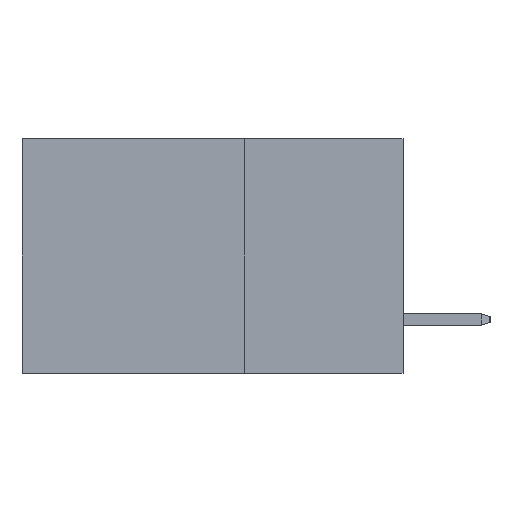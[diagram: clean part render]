
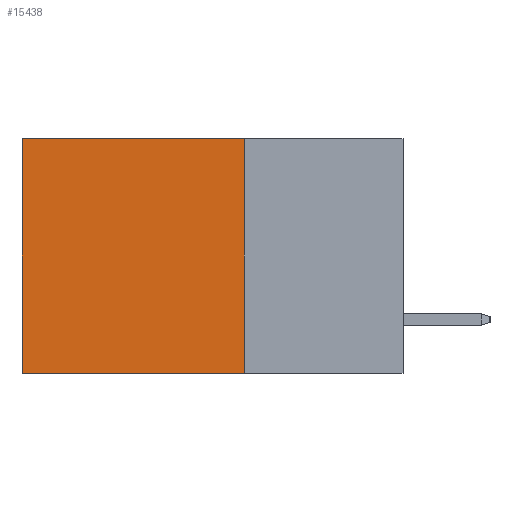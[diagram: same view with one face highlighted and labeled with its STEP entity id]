
A CAD part, left-side view. The second image highlights one B-rep face of the part: STEP entity #15438.
In plain terms, the highlighted planar face has unit normal (-1, 0, 0).
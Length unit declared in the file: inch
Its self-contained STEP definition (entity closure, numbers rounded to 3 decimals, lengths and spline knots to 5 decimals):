
#345 = VERTEX_POINT ( 'NONE', #10332 ) ;
#437 = DIRECTION ( 'NONE',  ( 0., 1., 0. ) ) ;
#1494 = CARTESIAN_POINT ( 'NONE',  ( 0.2875, 0.6, 0. ) ) ;
#1544 = CARTESIAN_POINT ( 'NONE',  ( 0.2875, 0.25, -0.37 ) ) ;
#1987 = VERTEX_POINT ( 'NONE', #7854 ) ;
#2152 = AXIS2_PLACEMENT_3D ( 'NONE', #7720, #12922, #12130 ) ;
#2515 = PLANE ( 'NONE',  #2152 ) ;
#2656 = VERTEX_POINT ( 'NONE', #9870 ) ;
#4456 = LINE ( 'NONE', #1544, #7580 ) ;
#4631 = EDGE_CURVE ( 'NONE', #1987, #2656, #4456, .T. ) ;
#4733 = EDGE_CURVE ( 'NONE', #345, #10092, #6666, .T. ) ;
#5535 = VECTOR ( 'NONE', #11903, 39.37008 ) ;
#5857 = DIRECTION ( 'NONE',  ( 0., 0., -1. ) ) ;
#5932 = EDGE_CURVE ( 'NONE', #345, #1987, #12083, .T. ) ;
#6666 = LINE ( 'NONE', #15775, #7291 ) ;
#7291 = VECTOR ( 'NONE', #8117, 39.37008 ) ;
#7580 = VECTOR ( 'NONE', #437, 39.37008 ) ;
#7720 = CARTESIAN_POINT ( 'NONE',  ( 0.2875, 0.25, 0. ) ) ;
#7854 = CARTESIAN_POINT ( 'NONE',  ( 0.2875, 0.25, -0.37 ) ) ;
#8117 = DIRECTION ( 'NONE',  ( 0., 1., 0. ) ) ;
#8419 = CARTESIAN_POINT ( 'NONE',  ( 0.2875, 0.25, 0. ) ) ;
#8992 = FACE_OUTER_BOUND ( 'NONE', #11119, .T. ) ;
#9450 = ORIENTED_EDGE ( 'NONE', *, *, #4733, .T. ) ;
#9870 = CARTESIAN_POINT ( 'NONE',  ( 0.2875, 0.6, -0.37 ) ) ;
#10092 = VERTEX_POINT ( 'NONE', #11497 ) ;
#10332 = CARTESIAN_POINT ( 'NONE',  ( 0.2875, 0.25, 0. ) ) ;
#11119 = EDGE_LOOP ( 'NONE', ( #16770, #13647, #13710, #9450 ) ) ;
#11497 = CARTESIAN_POINT ( 'NONE',  ( 0.2875, 0.6, 0. ) ) ;
#11903 = DIRECTION ( 'NONE',  ( 0., 0., -1. ) ) ;
#12083 = LINE ( 'NONE', #8419, #15204 ) ;
#12130 = DIRECTION ( 'NONE',  ( 0., 0., -1. ) ) ;
#12738 = EDGE_CURVE ( 'NONE', #10092, #2656, #12951, .T. ) ;
#12922 = DIRECTION ( 'NONE',  ( 1., 0., 0. ) ) ;
#12951 = LINE ( 'NONE', #1494, #5535 ) ;
#13647 = ORIENTED_EDGE ( 'NONE', *, *, #4631, .F. ) ;
#13710 = ORIENTED_EDGE ( 'NONE', *, *, #5932, .F. ) ;
#15204 = VECTOR ( 'NONE', #5857, 39.37008 ) ;
#15438 = ADVANCED_FACE ( 'NONE', ( #8992 ), #2515, .F. ) ;
#15775 = CARTESIAN_POINT ( 'NONE',  ( 0.2875, 0.25, 0. ) ) ;
#16770 = ORIENTED_EDGE ( 'NONE', *, *, #12738, .T. ) ;
